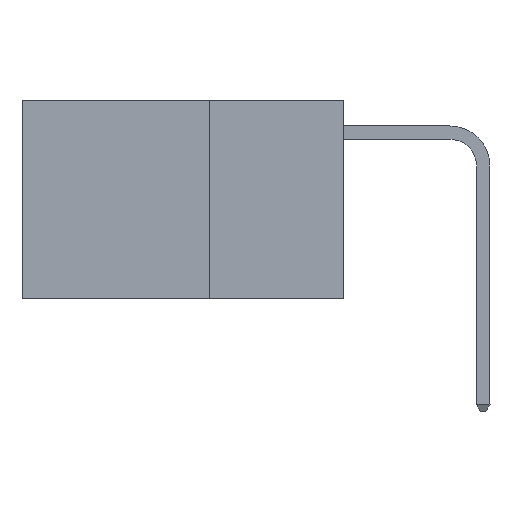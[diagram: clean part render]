
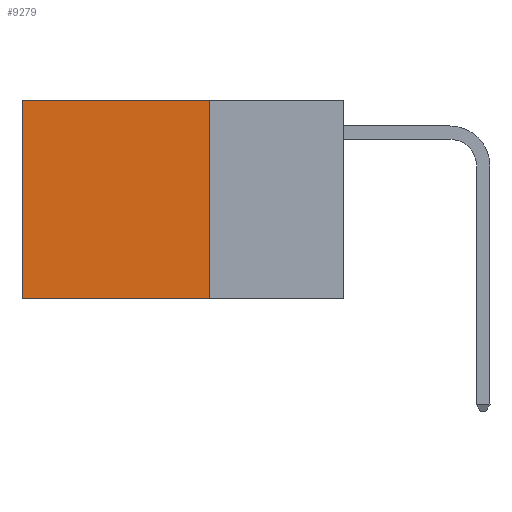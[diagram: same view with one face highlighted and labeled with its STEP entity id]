
A CAD part, left-side view. The second image highlights one B-rep face of the part: STEP entity #9279.
In plain terms, the highlighted planar face has unit normal (-1, 0, 0).
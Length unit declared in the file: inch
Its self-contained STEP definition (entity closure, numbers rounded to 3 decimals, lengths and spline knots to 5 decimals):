
#979 = LINE ( 'NONE', #1196, #11864 ) ;
#1196 = CARTESIAN_POINT ( 'NONE',  ( 0.2625, 0.25, 0. ) ) ;
#1223 = EDGE_CURVE ( 'NONE', #19274, #6457, #979, .T. ) ;
#1468 = EDGE_CURVE ( 'NONE', #10669, #15011, #2218, .T. ) ;
#1513 = EDGE_CURVE ( 'NONE', #19274, #10669, #6365, .T. ) ;
#2218 = LINE ( 'NONE', #9232, #9553 ) ;
#3982 = DIRECTION ( 'NONE',  ( 0., 0., -1. ) ) ;
#4420 = CARTESIAN_POINT ( 'NONE',  ( 0.2625, 0.25, 0. ) ) ;
#4975 = ORIENTED_EDGE ( 'NONE', *, *, #1468, .T. ) ;
#5311 = AXIS2_PLACEMENT_3D ( 'NONE', #6164, #17961, #3982 ) ;
#5924 = FACE_OUTER_BOUND ( 'NONE', #7460, .T. ) ;
#6164 = CARTESIAN_POINT ( 'NONE',  ( 0.2625, 0.25, 0. ) ) ;
#6365 = LINE ( 'NONE', #4420, #6994 ) ;
#6457 = VERTEX_POINT ( 'NONE', #8736 ) ;
#6503 = CARTESIAN_POINT ( 'NONE',  ( 0.2625, 0.25, 0. ) ) ;
#6713 = LINE ( 'NONE', #13783, #15400 ) ;
#6994 = VECTOR ( 'NONE', #18522, 39.37008 ) ;
#7460 = EDGE_LOOP ( 'NONE', ( #4975, #13014, #13891, #18854 ) ) ;
#8736 = CARTESIAN_POINT ( 'NONE',  ( 0.2625, 0.25, -0.37 ) ) ;
#9232 = CARTESIAN_POINT ( 'NONE',  ( 0.2625, 0.6, 0. ) ) ;
#9279 = ADVANCED_FACE ( 'NONE', ( #5924 ), #9377, .F. ) ;
#9377 = PLANE ( 'NONE',  #5311 ) ;
#9553 = VECTOR ( 'NONE', #12774, 39.37008 ) ;
#10669 = VERTEX_POINT ( 'NONE', #17155 ) ;
#11864 = VECTOR ( 'NONE', #13045, 39.37008 ) ;
#12774 = DIRECTION ( 'NONE',  ( 0., 0., -1. ) ) ;
#13014 = ORIENTED_EDGE ( 'NONE', *, *, #14627, .F. ) ;
#13045 = DIRECTION ( 'NONE',  ( 0., 0., -1. ) ) ;
#13783 = CARTESIAN_POINT ( 'NONE',  ( 0.2625, 0.25, -0.37 ) ) ;
#13891 = ORIENTED_EDGE ( 'NONE', *, *, #1223, .F. ) ;
#14627 = EDGE_CURVE ( 'NONE', #6457, #15011, #6713, .T. ) ;
#15011 = VERTEX_POINT ( 'NONE', #20437 ) ;
#15071 = DIRECTION ( 'NONE',  ( 0., 1., 0. ) ) ;
#15400 = VECTOR ( 'NONE', #15071, 39.37008 ) ;
#17155 = CARTESIAN_POINT ( 'NONE',  ( 0.2625, 0.6, 0. ) ) ;
#17961 = DIRECTION ( 'NONE',  ( 1., 0., 0. ) ) ;
#18522 = DIRECTION ( 'NONE',  ( 0., 1., 0. ) ) ;
#18854 = ORIENTED_EDGE ( 'NONE', *, *, #1513, .T. ) ;
#19274 = VERTEX_POINT ( 'NONE', #6503 ) ;
#20437 = CARTESIAN_POINT ( 'NONE',  ( 0.2625, 0.6, -0.37 ) ) ;
